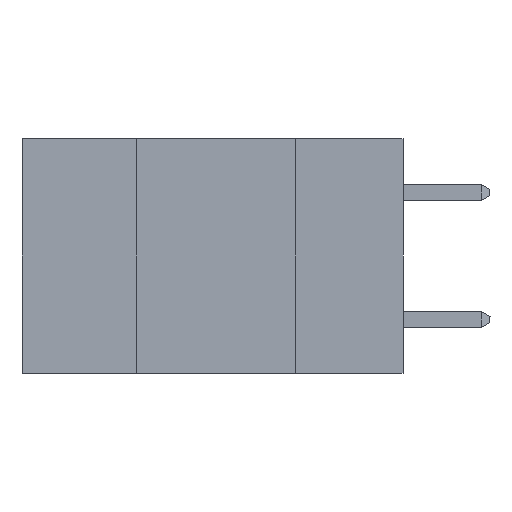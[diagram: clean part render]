
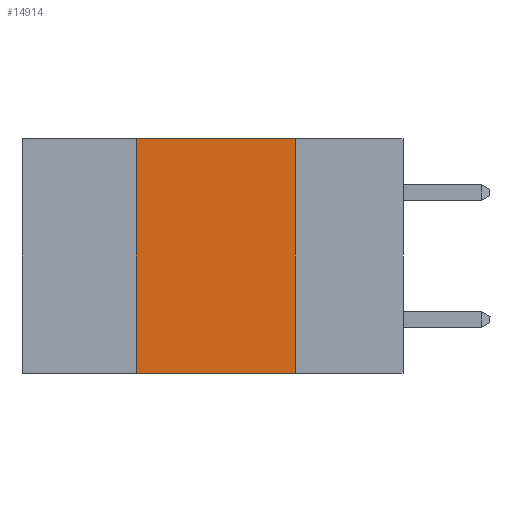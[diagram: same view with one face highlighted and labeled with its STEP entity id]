
A CAD part, left-side view. The second image highlights one B-rep face of the part: STEP entity #14914.
In plain terms, the highlighted planar face has unit normal (-1, 0, 0).
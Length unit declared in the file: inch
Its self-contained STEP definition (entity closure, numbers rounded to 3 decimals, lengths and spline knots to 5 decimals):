
#1627 = LINE ( 'NONE', #10236, #10212 ) ;
#2884 = CARTESIAN_POINT ( 'NONE',  ( 0., 0.17, -0.37 ) ) ;
#3301 = DIRECTION ( 'NONE',  ( 0., 0., -1. ) ) ;
#4120 = EDGE_LOOP ( 'NONE', ( #21696, #27515, #22789, #32664 ) ) ;
#4837 = CARTESIAN_POINT ( 'NONE',  ( 0., 0.6, -0.37 ) ) ;
#5202 = VECTOR ( 'NONE', #11023, 39.37008 ) ;
#7916 = EDGE_CURVE ( 'NONE', #25045, #35725, #18461, .T. ) ;
#8771 = CARTESIAN_POINT ( 'NONE',  ( 0., 0.42, 0. ) ) ;
#10212 = VECTOR ( 'NONE', #37561, 39.37008 ) ;
#10221 = EDGE_CURVE ( 'NONE', #34717, #25045, #32763, .T. ) ;
#10236 = CARTESIAN_POINT ( 'NONE',  ( 0., 0.42, 0. ) ) ;
#11023 = DIRECTION ( 'NONE',  ( 0., -1., 0. ) ) ;
#14914 = ADVANCED_FACE ( 'NONE', ( #33218 ), #33607, .F. ) ;
#14983 = CARTESIAN_POINT ( 'NONE',  ( 0., 0.6, 0. ) ) ;
#15218 = EDGE_CURVE ( 'NONE', #29757, #35725, #35352, .T. ) ;
#15246 = CARTESIAN_POINT ( 'NONE',  ( 0., 0.6, 0. ) ) ;
#17950 = AXIS2_PLACEMENT_3D ( 'NONE', #15246, #33409, #36207 ) ;
#18461 = LINE ( 'NONE', #30644, #38222 ) ;
#21696 = ORIENTED_EDGE ( 'NONE', *, *, #7916, .F. ) ;
#22789 = ORIENTED_EDGE ( 'NONE', *, *, #33376, .F. ) ;
#25045 = VERTEX_POINT ( 'NONE', #27105 ) ;
#27105 = CARTESIAN_POINT ( 'NONE',  ( 0., 0.17, 0. ) ) ;
#27515 = ORIENTED_EDGE ( 'NONE', *, *, #10221, .F. ) ;
#29757 = VERTEX_POINT ( 'NONE', #38766 ) ;
#30644 = CARTESIAN_POINT ( 'NONE',  ( 0., 0.17, 0. ) ) ;
#32664 = ORIENTED_EDGE ( 'NONE', *, *, #15218, .T. ) ;
#32763 = LINE ( 'NONE', #14983, #34290 ) ;
#33218 = FACE_OUTER_BOUND ( 'NONE', #4120, .T. ) ;
#33376 = EDGE_CURVE ( 'NONE', #29757, #34717, #1627, .T. ) ;
#33409 = DIRECTION ( 'NONE',  ( 1., 0., 0. ) ) ;
#33607 = PLANE ( 'NONE',  #17950 ) ;
#34290 = VECTOR ( 'NONE', #39338, 39.37008 ) ;
#34717 = VERTEX_POINT ( 'NONE', #8771 ) ;
#35352 = LINE ( 'NONE', #4837, #5202 ) ;
#35725 = VERTEX_POINT ( 'NONE', #2884 ) ;
#36207 = DIRECTION ( 'NONE',  ( 0., 0., -1. ) ) ;
#37561 = DIRECTION ( 'NONE',  ( 0., 0., 1. ) ) ;
#38222 = VECTOR ( 'NONE', #3301, 39.37008 ) ;
#38766 = CARTESIAN_POINT ( 'NONE',  ( 0., 0.42, -0.37 ) ) ;
#39338 = DIRECTION ( 'NONE',  ( 0., -1., 0. ) ) ;
